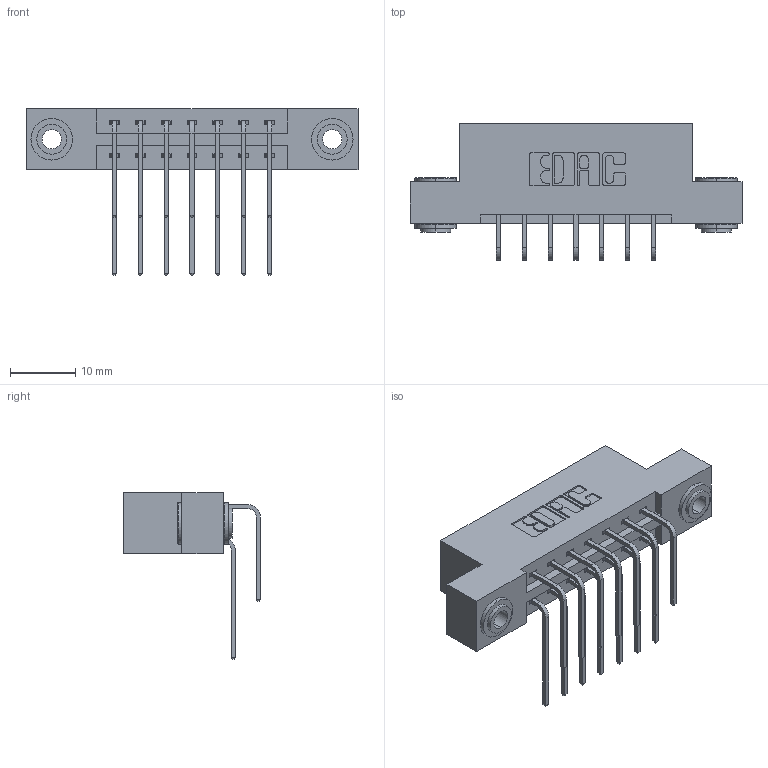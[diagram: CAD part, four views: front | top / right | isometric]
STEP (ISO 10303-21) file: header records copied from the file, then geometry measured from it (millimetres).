
FILE_DESCRIPTION (( 'STEP AP203' ), '1' );
FILE_NAME ('337-014-559-203.STEP', '2018-08-04T16:06:00', ( '' ), ( '' ), 'SwSTEP 2.0', 'SolidWorks 2016', '' );
FILE_SCHEMA (( 'CONFIG_CONTROL_DESIGN' ));
Length unit declared in the file: inch
Products named in the file (5): 337 Part_Flush Mounting Lugs - 0.156 Dia-TH; 345-292-001_558 559 Tail - 1; 345-292-001_559 Tail - 2; 345-250-002_345-250-002-102; 337-014-559-203
Assembly tree (17 placements, depth 2):
  337-014-559-203
    337 Part_Flush Mounting Lugs - 0.156 Dia-TH
    345-292-001_558 559 Tail - 1  x7
    345-292-001_559 Tail - 2  x7
    345-250-002_345-250-002-102  x2
Bounding box: 50.75 x 20.9 x 25.53 mm (x, y, z)
Volume: 4982.6 mm3; surface area: 5922.8 mm2
Topology: 17 solids, 17 shells, 936 faces, 2725 edges, 1794 vertices
Faces by surface type: plane 640, cylinder 288, cone 8
Entity records: 12388 total; most frequent: CARTESIAN_POINT 2136, ORIENTED_EDGE 2014, DIRECTION 1897, EDGE_CURVE 1007, LINE 815, VECTOR 815, VERTEX_POINT 666, AXIS2_PLACEMENT_3D 541
